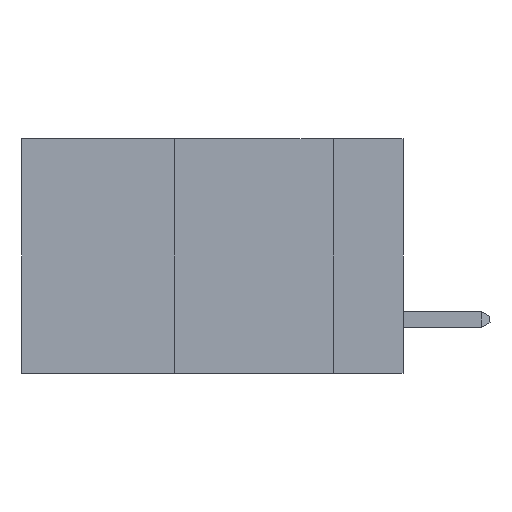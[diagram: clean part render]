
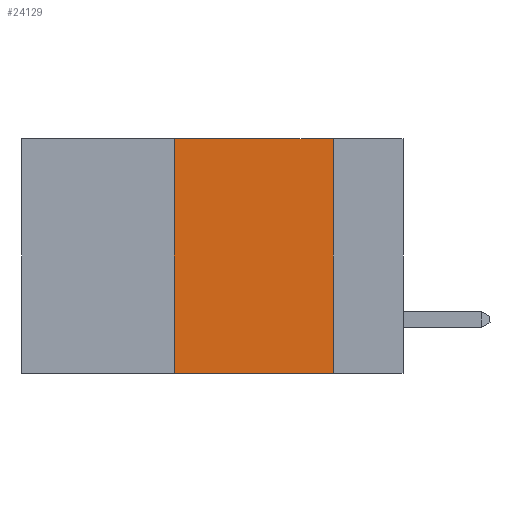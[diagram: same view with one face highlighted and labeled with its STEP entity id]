
A CAD part, left-side view. The second image highlights one B-rep face of the part: STEP entity #24129.
In plain terms, the highlighted planar face has unit normal (-1, 0, 0).
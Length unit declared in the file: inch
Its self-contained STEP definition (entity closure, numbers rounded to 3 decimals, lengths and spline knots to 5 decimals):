
#363 = CARTESIAN_POINT ( 'NONE',  ( 0., 0.6, -0.37 ) ) ;
#702 = VECTOR ( 'NONE', #17263, 39.37008 ) ;
#762 = EDGE_CURVE ( 'NONE', #23965, #14322, #9878, .T. ) ;
#954 = ORIENTED_EDGE ( 'NONE', *, *, #762, .F. ) ;
#1327 = EDGE_CURVE ( 'NONE', #20391, #23965, #24427, .T. ) ;
#3329 = DIRECTION ( 'NONE',  ( 1., 0., 0. ) ) ;
#3814 = VECTOR ( 'NONE', #13338, 39.37008 ) ;
#4096 = VECTOR ( 'NONE', #15263, 39.37008 ) ;
#6856 = VECTOR ( 'NONE', #16742, 39.37008 ) ;
#7392 = AXIS2_PLACEMENT_3D ( 'NONE', #26968, #3329, #18471 ) ;
#8748 = ORIENTED_EDGE ( 'NONE', *, *, #10429, .T. ) ;
#9603 = LINE ( 'NONE', #363, #3814 ) ;
#9878 = LINE ( 'NONE', #15953, #4096 ) ;
#10429 = EDGE_CURVE ( 'NONE', #20391, #24811, #9603, .T. ) ;
#10749 = CARTESIAN_POINT ( 'NONE',  ( 0., 0.36, -0.37 ) ) ;
#11797 = EDGE_LOOP ( 'NONE', ( #23318, #954, #18908, #8748 ) ) ;
#13338 = DIRECTION ( 'NONE',  ( 0., -1., 0. ) ) ;
#14322 = VERTEX_POINT ( 'NONE', #14598 ) ;
#14598 = CARTESIAN_POINT ( 'NONE',  ( 0., 0.11, 0. ) ) ;
#15263 = DIRECTION ( 'NONE',  ( 0., -1., 0. ) ) ;
#15953 = CARTESIAN_POINT ( 'NONE',  ( 0., 0.6, 0. ) ) ;
#16291 = PLANE ( 'NONE',  #7392 ) ;
#16742 = DIRECTION ( 'NONE',  ( 0., 0., -1. ) ) ;
#17263 = DIRECTION ( 'NONE',  ( 0., 0., 1. ) ) ;
#17712 = LINE ( 'NONE', #23290, #6856 ) ;
#18471 = DIRECTION ( 'NONE',  ( 0., 0., -1. ) ) ;
#18908 = ORIENTED_EDGE ( 'NONE', *, *, #1327, .F. ) ;
#19589 = FACE_OUTER_BOUND ( 'NONE', #11797, .T. ) ;
#20391 = VERTEX_POINT ( 'NONE', #10749 ) ;
#22183 = CARTESIAN_POINT ( 'NONE',  ( 0., 0.36, 0. ) ) ;
#22443 = EDGE_CURVE ( 'NONE', #14322, #24811, #17712, .T. ) ;
#23290 = CARTESIAN_POINT ( 'NONE',  ( 0., 0.11, 0. ) ) ;
#23318 = ORIENTED_EDGE ( 'NONE', *, *, #22443, .F. ) ;
#23707 = CARTESIAN_POINT ( 'NONE',  ( 0., 0.36, 0. ) ) ;
#23965 = VERTEX_POINT ( 'NONE', #22183 ) ;
#24129 = ADVANCED_FACE ( 'NONE', ( #19589 ), #16291, .F. ) ;
#24427 = LINE ( 'NONE', #23707, #702 ) ;
#24811 = VERTEX_POINT ( 'NONE', #24970 ) ;
#24970 = CARTESIAN_POINT ( 'NONE',  ( 0., 0.11, -0.37 ) ) ;
#26968 = CARTESIAN_POINT ( 'NONE',  ( 0., 0.6, 0. ) ) ;
